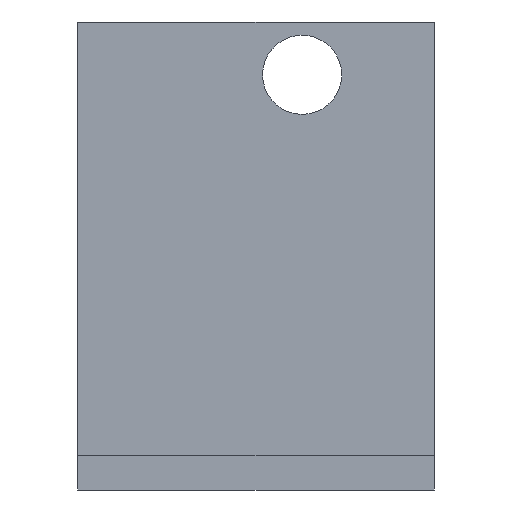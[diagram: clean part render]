
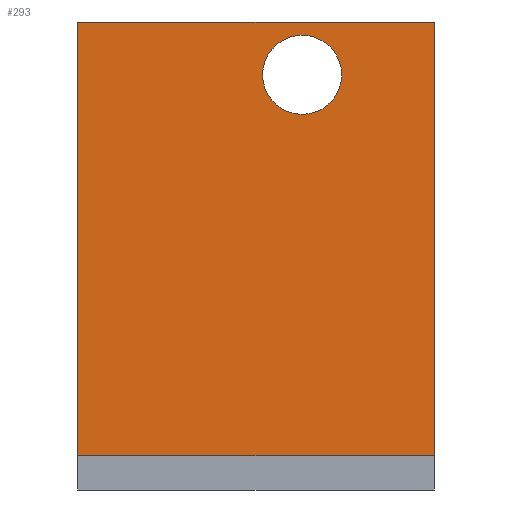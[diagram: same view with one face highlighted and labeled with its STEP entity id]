
A CAD part, front view. The second image highlights one B-rep face of the part: STEP entity #293.
In plain terms, the highlighted planar face has unit normal (0, -1, 0).
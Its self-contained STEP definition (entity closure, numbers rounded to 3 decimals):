
#15=FACE_BOUND('',#51,.T.);
#22=CIRCLE('',#324,1.5);
#35=FACE_OUTER_BOUND('',#50,.T.);
#50=EDGE_LOOP('',(#246,#247,#248,#249));
#51=EDGE_LOOP('',(#250));
#56=LINE('',#410,#91);
#66=LINE('',#431,#101);
#83=LINE('',#468,#118);
#88=LINE('',#481,#123);
#91=VECTOR('',#334,10.);
#101=VECTOR('',#350,10.);
#118=VECTOR('',#383,10.);
#123=VECTOR('',#398,10.);
#125=VERTEX_POINT('',#406);
#127=VERTEX_POINT('',#409);
#135=VERTEX_POINT('',#430);
#147=VERTEX_POINT('',#467);
#150=VERTEX_POINT('',#475);
#152=EDGE_CURVE('',#127,#125,#56,.T.);
#162=EDGE_CURVE('',#135,#125,#66,.T.);
#181=EDGE_CURVE('',#147,#135,#83,.T.);
#186=EDGE_CURVE('',#150,#150,#22,.T.);
#188=EDGE_CURVE('',#127,#147,#88,.T.);
#246=ORIENTED_EDGE('',*,*,#162,.F.);
#247=ORIENTED_EDGE('',*,*,#181,.F.);
#248=ORIENTED_EDGE('',*,*,#188,.F.);
#249=ORIENTED_EDGE('',*,*,#152,.T.);
#250=ORIENTED_EDGE('',*,*,#186,.F.);
#278=PLANE('',#326);
#293=ADVANCED_FACE('',(#35,#15),#278,.T.);
#324=AXIS2_PLACEMENT_3D('',#477,#391,#392);
#326=AXIS2_PLACEMENT_3D('',#480,#396,#397);
#334=DIRECTION('',(1.,0.,0.));
#350=DIRECTION('',(0.,0.,-1.));
#383=DIRECTION('',(1.,0.,0.));
#391=DIRECTION('center_axis',(0.,-1.,0.));
#392=DIRECTION('ref_axis',(1.,0.,0.));
#396=DIRECTION('center_axis',(0.,-1.,0.));
#397=DIRECTION('ref_axis',(0.,0.,-1.));
#398=DIRECTION('',(0.,0.,1.));
#406=CARTESIAN_POINT('',(31.329,-8.1,-29.184));
#409=CARTESIAN_POINT('',(17.829,-8.1,-29.184));
#410=CARTESIAN_POINT('',(16.829,-8.1,-29.184));
#430=CARTESIAN_POINT('',(31.329,-8.1,-12.75));
#431=CARTESIAN_POINT('',(31.329,-8.1,-14.75));
#467=CARTESIAN_POINT('',(17.829,-8.1,-12.75));
#468=CARTESIAN_POINT('',(17.329,-8.1,-12.75));
#475=CARTESIAN_POINT('',(24.829,-8.1,-14.75));
#477=CARTESIAN_POINT('Origin',(26.329,-8.1,-14.75));
#480=CARTESIAN_POINT('Origin',(16.829,-8.1,-14.75));
#481=CARTESIAN_POINT('',(17.829,-8.1,-21.637));
